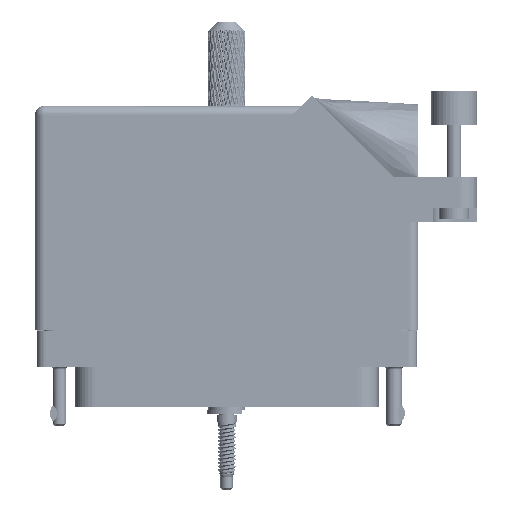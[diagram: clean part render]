
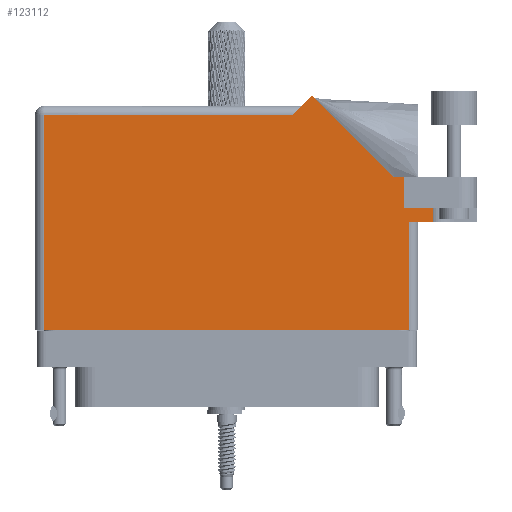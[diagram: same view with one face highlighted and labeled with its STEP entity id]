
A CAD part, front view. The second image highlights one B-rep face of the part: STEP entity #123112.
In plain terms, the highlighted face is planar.
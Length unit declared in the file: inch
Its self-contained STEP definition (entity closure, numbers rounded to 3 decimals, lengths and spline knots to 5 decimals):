
#883 = DIRECTION ( 'NONE',  ( -0.707, 0.707, 0. ) ) ;
#1330 = CARTESIAN_POINT ( 'NONE',  ( 1.306, 0.637, 0.455 ) ) ;
#1638 = LINE ( 'NONE', #27927, #101654 ) ;
#1671 = VERTEX_POINT ( 'NONE', #84414 ) ;
#2356 = VERTEX_POINT ( 'NONE', #36219 ) ;
#2929 = VERTEX_POINT ( 'NONE', #80348 ) ;
#6065 = VERTEX_POINT ( 'NONE', #66570 ) ;
#7119 = ORIENTED_EDGE ( 'NONE', *, *, #49473, .T. ) ;
#7418 = VECTOR ( 'NONE', #54108, 39.37008 ) ;
#7711 = VECTOR ( 'NONE', #122703, 39.37008 ) ;
#10794 = VECTOR ( 'NONE', #72510, 39.37008 ) ;
#11475 = EDGE_CURVE ( 'NONE', #103101, #2929, #1638, .T. ) ;
#12346 = FACE_OUTER_BOUND ( 'NONE', #21419, .T. ) ;
#13901 = EDGE_CURVE ( 'NONE', #44897, #30962, #67317, .T. ) ;
#15583 = VERTEX_POINT ( 'NONE', #31939 ) ;
#15801 = LINE ( 'NONE', #120753, #49601 ) ;
#19813 = CARTESIAN_POINT ( 'NONE',  ( 1.4075, 0.731, 0.455 ) ) ;
#21419 = EDGE_LOOP ( 'NONE', ( #54913, #29112, #36256, #40128, #112503, #29952, #103743, #68639, #88648, #7119, #58468 ) ) ;
#23015 = VECTOR ( 'NONE', #124675, 39.37008 ) ;
#23382 = EDGE_CURVE ( 'NONE', #1671, #103101, #97991, .T. ) ;
#24028 = VECTOR ( 'NONE', #64274, 39.37008 ) ;
#25175 = CARTESIAN_POINT ( 'NONE',  ( 1.244, 0.637, 0.455 ) ) ;
#27927 = CARTESIAN_POINT ( 'NONE',  ( 1.14042, 0.944, 0.455 ) ) ;
#29112 = ORIENTED_EDGE ( 'NONE', *, *, #65418, .T. ) ;
#29952 = ORIENTED_EDGE ( 'NONE', *, *, #75433, .T. ) ;
#30962 = VERTEX_POINT ( 'NONE', #95676 ) ;
#31191 = LINE ( 'NONE', #63882, #98919 ) ;
#31836 = CARTESIAN_POINT ( 'NONE',  ( -1.244, -0.1, 0.455 ) ) ;
#31886 = VERTEX_POINT ( 'NONE', #19813 ) ;
#31939 = CARTESIAN_POINT ( 'NONE',  ( 1.244, -0.1, 0.455 ) ) ;
#32519 = CARTESIAN_POINT ( 'NONE',  ( 1.206, 0.731, 0.455 ) ) ;
#33529 = DIRECTION ( 'NONE',  ( -0.707, -0.707, 0. ) ) ;
#34158 = DIRECTION ( 'NONE',  ( -1., 0., 0. ) ) ;
#36219 = CARTESIAN_POINT ( 'NONE',  ( 0.451, 1.368, 0.455 ) ) ;
#36256 = ORIENTED_EDGE ( 'NONE', *, *, #125647, .T. ) ;
#40128 = ORIENTED_EDGE ( 'NONE', *, *, #42525, .F. ) ;
#40468 = DIRECTION ( 'NONE',  ( -1., 0., 0. ) ) ;
#42525 = EDGE_CURVE ( 'NONE', #31886, #6065, #69116, .T. ) ;
#44897 = VERTEX_POINT ( 'NONE', #80805 ) ;
#49137 = CARTESIAN_POINT ( 'NONE',  ( -1.306, 1.43, 0.455 ) ) ;
#49473 = EDGE_CURVE ( 'NONE', #2356, #44897, #106153, .T. ) ;
#49601 = VECTOR ( 'NONE', #33529, 39.37008 ) ;
#50204 = LINE ( 'NONE', #25175, #24028 ) ;
#54108 = DIRECTION ( 'NONE',  ( 0., -1., 0. ) ) ;
#54913 = ORIENTED_EDGE ( 'NONE', *, *, #59989, .T. ) ;
#55901 = CARTESIAN_POINT ( 'NONE',  ( 1.4075, 1.06177, 0.455 ) ) ;
#58468 = ORIENTED_EDGE ( 'NONE', *, *, #13901, .T. ) ;
#59437 = EDGE_CURVE ( 'NONE', #59734, #31886, #31191, .T. ) ;
#59734 = VERTEX_POINT ( 'NONE', #32519 ) ;
#59989 = EDGE_CURVE ( 'NONE', #30962, #15583, #121812, .T. ) ;
#62892 = CARTESIAN_POINT ( 'NONE',  ( 1.706, 0.944, 0.455 ) ) ;
#63866 = CARTESIAN_POINT ( 'NONE',  ( -1.306, 1.368, 0.455 ) ) ;
#63882 = CARTESIAN_POINT ( 'NONE',  ( 1.206, 0.731, 0.455 ) ) ;
#64274 = DIRECTION ( 'NONE',  ( 0., 1., 0. ) ) ;
#65120 = CARTESIAN_POINT ( 'NONE',  ( 1.206, 0.731, 0.455 ) ) ;
#65418 = EDGE_CURVE ( 'NONE', #15583, #83258, #50204, .T. ) ;
#66570 = CARTESIAN_POINT ( 'NONE',  ( 1.4075, 0.637, 0.455 ) ) ;
#67317 = LINE ( 'NONE', #31836, #7418 ) ;
#68639 = ORIENTED_EDGE ( 'NONE', *, *, #11475, .T. ) ;
#69116 = LINE ( 'NONE', #55901, #23015 ) ;
#70661 = LINE ( 'NONE', #65120, #7711 ) ;
#71781 = VECTOR ( 'NONE', #34158, 39.37008 ) ;
#72510 = DIRECTION ( 'NONE',  ( -1., 0., 0. ) ) ;
#72769 = EDGE_CURVE ( 'NONE', #2929, #2356, #15801, .T. ) ;
#75433 = EDGE_CURVE ( 'NONE', #59734, #1671, #70661, .T. ) ;
#77175 = VECTOR ( 'NONE', #89077, 39.37008 ) ;
#78630 = DIRECTION ( 'NONE',  ( 1., 0., 0. ) ) ;
#79126 = PLANE ( 'NONE',  #109148 ) ;
#79530 = DIRECTION ( 'NONE',  ( 0., 0., -1. ) ) ;
#80348 = CARTESIAN_POINT ( 'NONE',  ( 0.58371, 1.50071, 0.455 ) ) ;
#80642 = CARTESIAN_POINT ( 'NONE',  ( 1.244, 0.637, 0.455 ) ) ;
#80805 = CARTESIAN_POINT ( 'NONE',  ( -1.244, 1.368, 0.455 ) ) ;
#83258 = VERTEX_POINT ( 'NONE', #80642 ) ;
#84414 = CARTESIAN_POINT ( 'NONE',  ( 1.206, 0.944, 0.455 ) ) ;
#88648 = ORIENTED_EDGE ( 'NONE', *, *, #72769, .T. ) ;
#89077 = DIRECTION ( 'NONE',  ( 1., 0., 0. ) ) ;
#93158 = DIRECTION ( 'NONE',  ( 1., 0., 0. ) ) ;
#95676 = CARTESIAN_POINT ( 'NONE',  ( -1.244, -0.1, 0.455 ) ) ;
#97991 = LINE ( 'NONE', #62892, #71781 ) ;
#98919 = VECTOR ( 'NONE', #93158, 39.37008 ) ;
#100041 = CARTESIAN_POINT ( 'NONE',  ( 1.14042, 0.944, 0.455 ) ) ;
#101654 = VECTOR ( 'NONE', #883, 39.37008 ) ;
#102611 = VECTOR ( 'NONE', #78630, 39.37008 ) ;
#103101 = VERTEX_POINT ( 'NONE', #100041 ) ;
#103743 = ORIENTED_EDGE ( 'NONE', *, *, #23382, .T. ) ;
#106153 = LINE ( 'NONE', #63866, #10794 ) ;
#108470 = CARTESIAN_POINT ( 'NONE',  ( -1.306, -0.1, 0.455 ) ) ;
#109148 = AXIS2_PLACEMENT_3D ( 'NONE', #49137, #79530, #40468 ) ;
#112503 = ORIENTED_EDGE ( 'NONE', *, *, #59437, .F. ) ;
#120753 = CARTESIAN_POINT ( 'NONE',  ( 0.513, 1.43, 0.455 ) ) ;
#121812 = LINE ( 'NONE', #108470, #77175 ) ;
#122544 = LINE ( 'NONE', #1330, #102611 ) ;
#122703 = DIRECTION ( 'NONE',  ( 0., 1., 0. ) ) ;
#123112 = ADVANCED_FACE ( 'NONE', ( #12346 ), #79126, .F. ) ;
#124675 = DIRECTION ( 'NONE',  ( 0., -1., 0. ) ) ;
#125647 = EDGE_CURVE ( 'NONE', #83258, #6065, #122544, .T. ) ;
